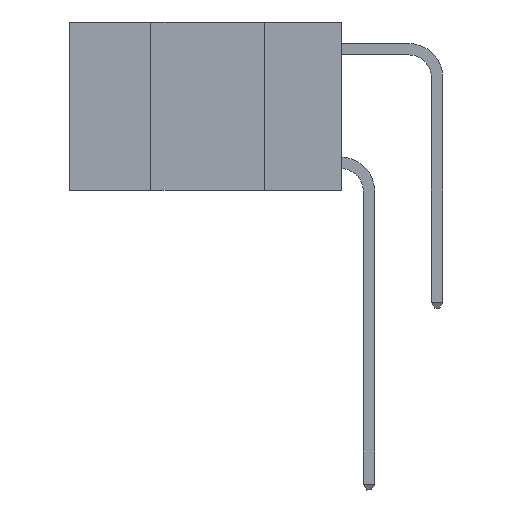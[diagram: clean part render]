
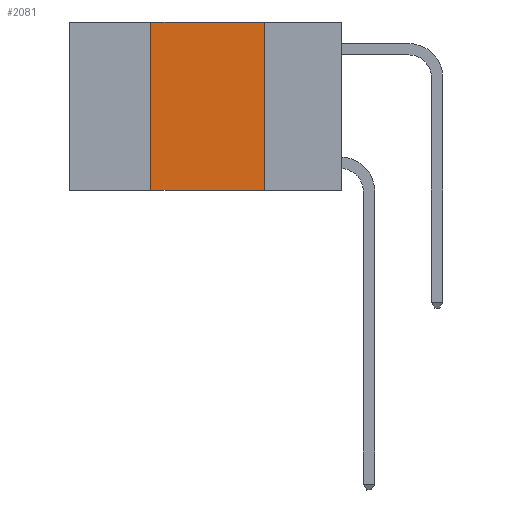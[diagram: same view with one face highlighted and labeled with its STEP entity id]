
A CAD part, left-side view. The second image highlights one B-rep face of the part: STEP entity #2081.
In plain terms, the highlighted planar face has unit normal (-1, 0, 0).
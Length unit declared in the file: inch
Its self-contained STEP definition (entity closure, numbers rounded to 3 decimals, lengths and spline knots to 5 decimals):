
#440 = EDGE_LOOP ( 'NONE', ( #15392, #13008, #1700, #9174 ) ) ;
#1241 = LINE ( 'NONE', #8262, #8172 ) ;
#1700 = ORIENTED_EDGE ( 'NONE', *, *, #9376, .F. ) ;
#1827 = CARTESIAN_POINT ( 'NONE',  ( 0., 0.6, -0.37 ) ) ;
#1855 = FACE_OUTER_BOUND ( 'NONE', #440, .T. ) ;
#2019 = VECTOR ( 'NONE', #8303, 39.37008 ) ;
#2081 = ADVANCED_FACE ( 'NONE', ( #1855 ), #15497, .F. ) ;
#3183 = DIRECTION ( 'NONE',  ( 0., -1., 0. ) ) ;
#3267 = LINE ( 'NONE', #1827, #12279 ) ;
#4373 = LINE ( 'NONE', #7309, #2019 ) ;
#4484 = DIRECTION ( 'NONE',  ( 0., 0., -1. ) ) ;
#5282 = AXIS2_PLACEMENT_3D ( 'NONE', #7423, #11219, #4484 ) ;
#5704 = DIRECTION ( 'NONE',  ( 0., -1., 0. ) ) ;
#5846 = EDGE_CURVE ( 'NONE', #13264, #6194, #17953, .T. ) ;
#6194 = VERTEX_POINT ( 'NONE', #12113 ) ;
#6893 = EDGE_CURVE ( 'NONE', #14532, #13721, #3267, .T. ) ;
#7309 = CARTESIAN_POINT ( 'NONE',  ( 0., 0.42, 0. ) ) ;
#7423 = CARTESIAN_POINT ( 'NONE',  ( 0., 0.6, 0. ) ) ;
#8172 = VECTOR ( 'NONE', #14037, 39.37008 ) ;
#8262 = CARTESIAN_POINT ( 'NONE',  ( 0., 0.17, 0. ) ) ;
#8303 = DIRECTION ( 'NONE',  ( 0., 0., 1. ) ) ;
#9174 = ORIENTED_EDGE ( 'NONE', *, *, #6893, .T. ) ;
#9376 = EDGE_CURVE ( 'NONE', #14532, #13264, #4373, .T. ) ;
#10371 = CARTESIAN_POINT ( 'NONE',  ( 0., 0.42, 0. ) ) ;
#11167 = EDGE_CURVE ( 'NONE', #6194, #13721, #1241, .T. ) ;
#11219 = DIRECTION ( 'NONE',  ( 1., 0., 0. ) ) ;
#12113 = CARTESIAN_POINT ( 'NONE',  ( 0., 0.17, 0. ) ) ;
#12279 = VECTOR ( 'NONE', #3183, 39.37008 ) ;
#13008 = ORIENTED_EDGE ( 'NONE', *, *, #5846, .F. ) ;
#13264 = VERTEX_POINT ( 'NONE', #10371 ) ;
#13721 = VERTEX_POINT ( 'NONE', #16430 ) ;
#13874 = CARTESIAN_POINT ( 'NONE',  ( 0., 0.6, 0. ) ) ;
#14037 = DIRECTION ( 'NONE',  ( 0., 0., -1. ) ) ;
#14532 = VERTEX_POINT ( 'NONE', #14553 ) ;
#14553 = CARTESIAN_POINT ( 'NONE',  ( 0., 0.42, -0.37 ) ) ;
#15392 = ORIENTED_EDGE ( 'NONE', *, *, #11167, .F. ) ;
#15497 = PLANE ( 'NONE',  #5282 ) ;
#15959 = VECTOR ( 'NONE', #5704, 39.37008 ) ;
#16430 = CARTESIAN_POINT ( 'NONE',  ( 0., 0.17, -0.37 ) ) ;
#17953 = LINE ( 'NONE', #13874, #15959 ) ;
